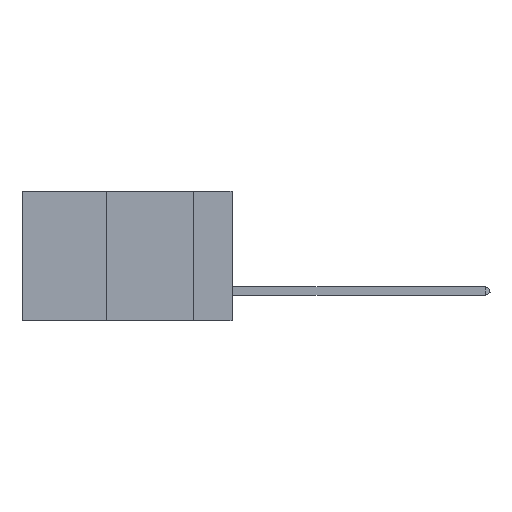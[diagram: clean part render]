
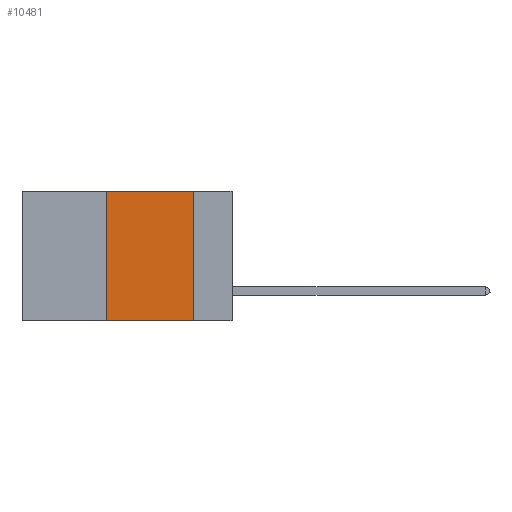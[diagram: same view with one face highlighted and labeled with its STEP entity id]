
A CAD part, left-side view. The second image highlights one B-rep face of the part: STEP entity #10481.
In plain terms, the highlighted planar face has unit normal (-1, 0, 0).
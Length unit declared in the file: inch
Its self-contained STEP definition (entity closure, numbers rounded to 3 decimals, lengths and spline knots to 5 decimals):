
#307 = CARTESIAN_POINT ( 'NONE',  ( 0., 0.36, 0. ) ) ;
#819 = VERTEX_POINT ( 'NONE', #13387 ) ;
#850 = CARTESIAN_POINT ( 'NONE',  ( 0., 0.11, -0.37 ) ) ;
#1106 = CARTESIAN_POINT ( 'NONE',  ( 0., 0.11, 0. ) ) ;
#1275 = VECTOR ( 'NONE', #2546, 39.37008 ) ;
#1664 = EDGE_CURVE ( 'NONE', #13487, #14289, #6275, .T. ) ;
#2409 = CARTESIAN_POINT ( 'NONE',  ( 0., 0.36, -0.37 ) ) ;
#2546 = DIRECTION ( 'NONE',  ( 0., 0., 1. ) ) ;
#2952 = VECTOR ( 'NONE', #5492, 39.37008 ) ;
#3958 = ORIENTED_EDGE ( 'NONE', *, *, #5190, .F. ) ;
#4177 = EDGE_LOOP ( 'NONE', ( #6806, #10501, #3958, #9213 ) ) ;
#4823 = VECTOR ( 'NONE', #6537, 39.37008 ) ;
#5190 = EDGE_CURVE ( 'NONE', #13487, #819, #5989, .T. ) ;
#5194 = VERTEX_POINT ( 'NONE', #7453 ) ;
#5492 = DIRECTION ( 'NONE',  ( 0., -1., 0. ) ) ;
#5613 = FACE_OUTER_BOUND ( 'NONE', #4177, .T. ) ;
#5989 = LINE ( 'NONE', #307, #1275 ) ;
#6275 = LINE ( 'NONE', #12319, #2952 ) ;
#6489 = AXIS2_PLACEMENT_3D ( 'NONE', #9719, #7371, #7419 ) ;
#6537 = DIRECTION ( 'NONE',  ( 0., -1., 0. ) ) ;
#6806 = ORIENTED_EDGE ( 'NONE', *, *, #13245, .F. ) ;
#7371 = DIRECTION ( 'NONE',  ( 1., 0., 0. ) ) ;
#7419 = DIRECTION ( 'NONE',  ( 0., 0., -1. ) ) ;
#7453 = CARTESIAN_POINT ( 'NONE',  ( 0., 0.11, 0. ) ) ;
#7751 = PLANE ( 'NONE',  #6489 ) ;
#9007 = LINE ( 'NONE', #13167, #4823 ) ;
#9213 = ORIENTED_EDGE ( 'NONE', *, *, #1664, .T. ) ;
#9719 = CARTESIAN_POINT ( 'NONE',  ( 0., 0.6, 0. ) ) ;
#9765 = DIRECTION ( 'NONE',  ( 0., 0., -1. ) ) ;
#10481 = ADVANCED_FACE ( 'NONE', ( #5613 ), #7751, .F. ) ;
#10501 = ORIENTED_EDGE ( 'NONE', *, *, #13900, .F. ) ;
#11987 = VECTOR ( 'NONE', #9765, 39.37008 ) ;
#12319 = CARTESIAN_POINT ( 'NONE',  ( 0., 0.6, -0.37 ) ) ;
#13008 = LINE ( 'NONE', #1106, #11987 ) ;
#13167 = CARTESIAN_POINT ( 'NONE',  ( 0., 0.6, 0. ) ) ;
#13245 = EDGE_CURVE ( 'NONE', #5194, #14289, #13008, .T. ) ;
#13387 = CARTESIAN_POINT ( 'NONE',  ( 0., 0.36, 0. ) ) ;
#13487 = VERTEX_POINT ( 'NONE', #2409 ) ;
#13900 = EDGE_CURVE ( 'NONE', #819, #5194, #9007, .T. ) ;
#14289 = VERTEX_POINT ( 'NONE', #850 ) ;
